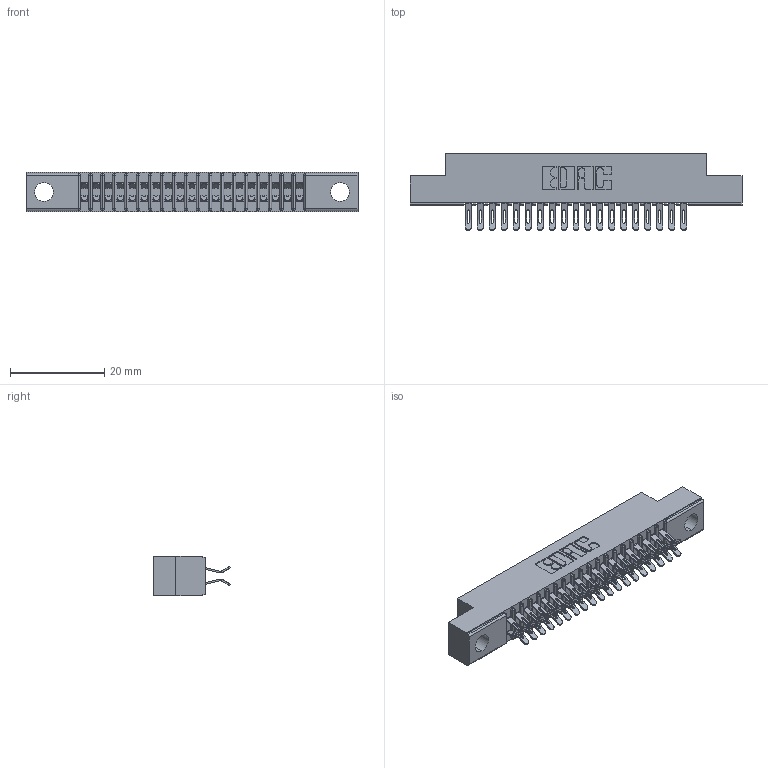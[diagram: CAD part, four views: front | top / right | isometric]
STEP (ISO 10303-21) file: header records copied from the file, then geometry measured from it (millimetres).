
FILE_DESCRIPTION (( 'STEP AP203' ), '1' );
FILE_NAME ('341-038-555-204.STEP', '2018-08-06T23:41:17', ( '' ), ( '' ), 'SwSTEP 2.0', 'SolidWorks 2016', '' );
FILE_SCHEMA (( 'CONFIG_CONTROL_DESIGN' ));
Length unit declared in the file: inch
Products named in the file (3): 341 Part_.156 (3.96) Dia Mounting Holes; 341-292-001_341-292-155; 341-038-555-204
Assembly tree (39 placements, depth 2):
  341-038-555-204
    341 Part_.156 (3.96) Dia Mounting Holes
    341-292-001_341-292-155  x38
Bounding box: 70.48 x 16.31 x 8.38 mm (x, y, z)
Volume: 3963.3 mm3; surface area: 8284.2 mm2
Topology: 39 solids, 39 shells, 3094 faces, 9225 edges, 6006 vertices
Faces by surface type: plane 1678, cylinder 1340, sphere 40, torus 36
Entity records: 26946 total; most frequent: CARTESIAN_POINT 4501, ORIENTED_EDGE 4458, DIRECTION 4367, EDGE_CURVE 2229, LINE 1767, VECTOR 1767, VERTEX_POINT 1418, AXIS2_PLACEMENT_3D 1300
